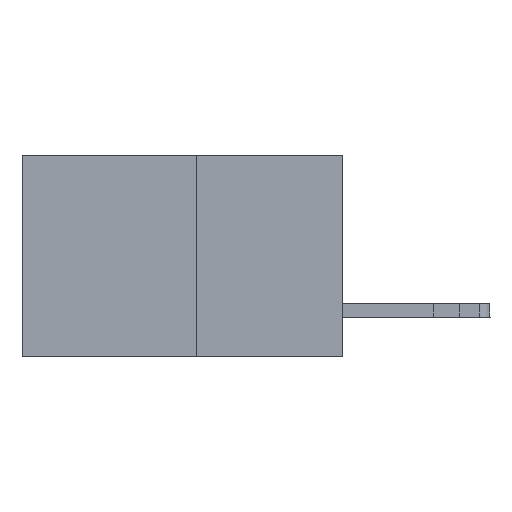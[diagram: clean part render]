
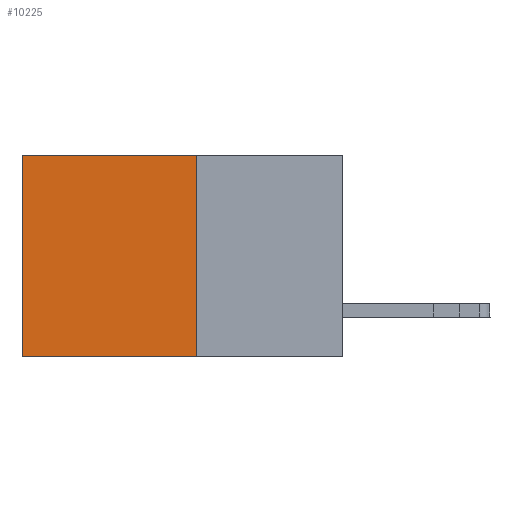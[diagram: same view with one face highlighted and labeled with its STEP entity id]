
A CAD part, left-side view. The second image highlights one B-rep face of the part: STEP entity #10225.
In plain terms, the highlighted planar face has unit normal (-1, 0, 0).
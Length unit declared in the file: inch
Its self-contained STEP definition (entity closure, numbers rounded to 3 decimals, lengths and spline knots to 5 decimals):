
#400 = LINE ( 'NONE', #12993, #6487 ) ;
#410 = CARTESIAN_POINT ( 'NONE',  ( 0.277, 0.59, -0.37 ) ) ;
#484 = ORIENTED_EDGE ( 'NONE', *, *, #12849, .F. ) ;
#729 = CARTESIAN_POINT ( 'NONE',  ( 0.277, 0.27, -0.37 ) ) ;
#2006 = VERTEX_POINT ( 'NONE', #12055 ) ;
#4053 = ORIENTED_EDGE ( 'NONE', *, *, #13735, .F. ) ;
#5097 = VECTOR ( 'NONE', #10139, 39.37008 ) ;
#5567 = DIRECTION ( 'NONE',  ( 0., 0., -1. ) ) ;
#5582 = CARTESIAN_POINT ( 'NONE',  ( 0.277, 0.27, 0. ) ) ;
#5896 = DIRECTION ( 'NONE',  ( 1., 0., 0. ) ) ;
#6487 = VECTOR ( 'NONE', #8315, 39.37008 ) ;
#6527 = DIRECTION ( 'NONE',  ( 0., 0., -1. ) ) ;
#7194 = VERTEX_POINT ( 'NONE', #729 ) ;
#7266 = LINE ( 'NONE', #12776, #10122 ) ;
#7635 = VERTEX_POINT ( 'NONE', #13170 ) ;
#8069 = AXIS2_PLACEMENT_3D ( 'NONE', #11865, #5896, #14133 ) ;
#8315 = DIRECTION ( 'NONE',  ( 0., 1., 0. ) ) ;
#8899 = CARTESIAN_POINT ( 'NONE',  ( 0.277, 0.27, -0.37 ) ) ;
#9968 = ORIENTED_EDGE ( 'NONE', *, *, #12526, .T. ) ;
#10122 = VECTOR ( 'NONE', #5567, 39.37008 ) ;
#10139 = DIRECTION ( 'NONE',  ( 0., 1., 0. ) ) ;
#10225 = ADVANCED_FACE ( 'NONE', ( #14603 ), #13072, .F. ) ;
#11030 = VECTOR ( 'NONE', #6527, 39.37008 ) ;
#11626 = LINE ( 'NONE', #8899, #5097 ) ;
#11865 = CARTESIAN_POINT ( 'NONE',  ( 0.277, 0.27, -0.37 ) ) ;
#11988 = ORIENTED_EDGE ( 'NONE', *, *, #14287, .T. ) ;
#12055 = CARTESIAN_POINT ( 'NONE',  ( 0.277, 0.59, -0.37 ) ) ;
#12526 = EDGE_CURVE ( 'NONE', #13054, #7635, #400, .T. ) ;
#12776 = CARTESIAN_POINT ( 'NONE',  ( 0.277, 0.27, -0.37 ) ) ;
#12849 = EDGE_CURVE ( 'NONE', #7194, #2006, #11626, .T. ) ;
#12993 = CARTESIAN_POINT ( 'NONE',  ( 0.277, 0.27, 0. ) ) ;
#13054 = VERTEX_POINT ( 'NONE', #5582 ) ;
#13072 = PLANE ( 'NONE',  #8069 ) ;
#13170 = CARTESIAN_POINT ( 'NONE',  ( 0.277, 0.59, 0. ) ) ;
#13735 = EDGE_CURVE ( 'NONE', #13054, #7194, #7266, .T. ) ;
#13956 = LINE ( 'NONE', #410, #11030 ) ;
#14133 = DIRECTION ( 'NONE',  ( 0., 0., -1. ) ) ;
#14287 = EDGE_CURVE ( 'NONE', #7635, #2006, #13956, .T. ) ;
#14603 = FACE_OUTER_BOUND ( 'NONE', #14747, .T. ) ;
#14747 = EDGE_LOOP ( 'NONE', ( #11988, #484, #4053, #9968 ) ) ;
